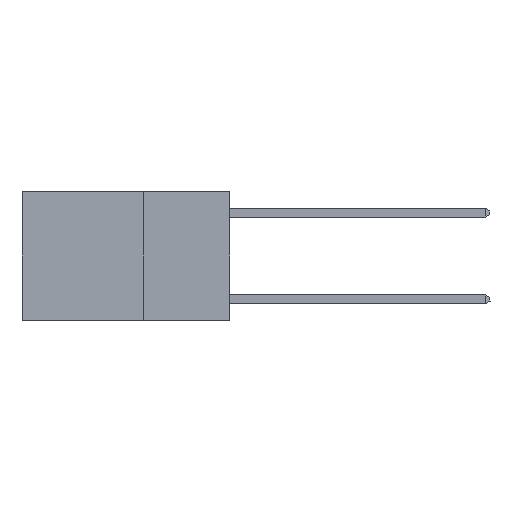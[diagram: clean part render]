
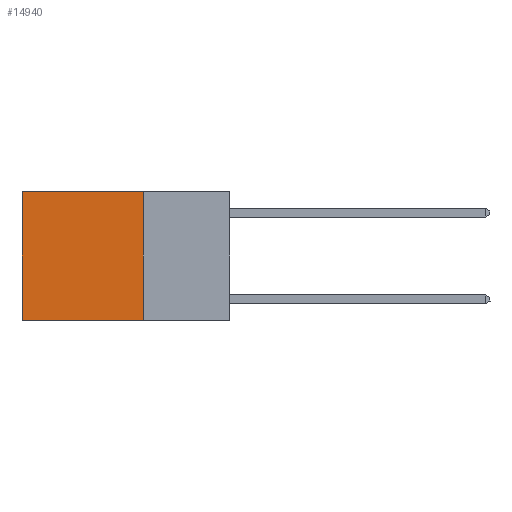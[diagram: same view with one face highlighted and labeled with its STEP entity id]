
A CAD part, left-side view. The second image highlights one B-rep face of the part: STEP entity #14940.
In plain terms, the highlighted planar face has unit normal (-1, 0, 0).
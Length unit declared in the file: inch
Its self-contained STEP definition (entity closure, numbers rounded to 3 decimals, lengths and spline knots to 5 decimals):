
#131 = DIRECTION ( 'NONE',  ( 0., 0., -1. ) ) ;
#175 = LINE ( 'NONE', #6093, #15766 ) ;
#477 = VERTEX_POINT ( 'NONE', #1827 ) ;
#612 = ORIENTED_EDGE ( 'NONE', *, *, #12786, .T. ) ;
#973 = DIRECTION ( 'NONE',  ( 0., 1., 0. ) ) ;
#1018 = CARTESIAN_POINT ( 'NONE',  ( 0.2625, 0.25, -0.37 ) ) ;
#1827 = CARTESIAN_POINT ( 'NONE',  ( 0.2625, 0.25, -0.37 ) ) ;
#1903 = CARTESIAN_POINT ( 'NONE',  ( 0.2625, 0.6, -0.37 ) ) ;
#3282 = VECTOR ( 'NONE', #8461, 39.37008 ) ;
#5583 = VECTOR ( 'NONE', #12988, 39.37008 ) ;
#6093 = CARTESIAN_POINT ( 'NONE',  ( 0.2625, 0.6, 0. ) ) ;
#6351 = LINE ( 'NONE', #17217, #3282 ) ;
#6955 = CARTESIAN_POINT ( 'NONE',  ( 0.2625, 0.25, 0. ) ) ;
#7615 = EDGE_CURVE ( 'NONE', #17538, #12568, #175, .T. ) ;
#8390 = FACE_OUTER_BOUND ( 'NONE', #15947, .T. ) ;
#8461 = DIRECTION ( 'NONE',  ( 0., 0., -1. ) ) ;
#9144 = DIRECTION ( 'NONE',  ( 1., 0., 0. ) ) ;
#10558 = DIRECTION ( 'NONE',  ( 0., 0., -1. ) ) ;
#11125 = AXIS2_PLACEMENT_3D ( 'NONE', #17877, #9144, #131 ) ;
#11266 = CARTESIAN_POINT ( 'NONE',  ( 0.2625, 0.6, 0. ) ) ;
#12539 = CARTESIAN_POINT ( 'NONE',  ( 0.2625, 0.25, 0. ) ) ;
#12568 = VERTEX_POINT ( 'NONE', #1903 ) ;
#12767 = EDGE_CURVE ( 'NONE', #13908, #477, #6351, .T. ) ;
#12786 = EDGE_CURVE ( 'NONE', #13908, #17538, #17582, .T. ) ;
#12988 = DIRECTION ( 'NONE',  ( 0., 1., 0. ) ) ;
#13308 = ORIENTED_EDGE ( 'NONE', *, *, #14676, .F. ) ;
#13735 = VECTOR ( 'NONE', #973, 39.37008 ) ;
#13801 = ORIENTED_EDGE ( 'NONE', *, *, #12767, .F. ) ;
#13908 = VERTEX_POINT ( 'NONE', #12539 ) ;
#14676 = EDGE_CURVE ( 'NONE', #477, #12568, #16399, .T. ) ;
#14940 = ADVANCED_FACE ( 'NONE', ( #8390 ), #14955, .F. ) ;
#14955 = PLANE ( 'NONE',  #11125 ) ;
#15617 = ORIENTED_EDGE ( 'NONE', *, *, #7615, .T. ) ;
#15766 = VECTOR ( 'NONE', #10558, 39.37008 ) ;
#15947 = EDGE_LOOP ( 'NONE', ( #15617, #13308, #13801, #612 ) ) ;
#16399 = LINE ( 'NONE', #1018, #5583 ) ;
#17217 = CARTESIAN_POINT ( 'NONE',  ( 0.2625, 0.25, 0. ) ) ;
#17538 = VERTEX_POINT ( 'NONE', #11266 ) ;
#17582 = LINE ( 'NONE', #6955, #13735 ) ;
#17877 = CARTESIAN_POINT ( 'NONE',  ( 0.2625, 0.25, 0. ) ) ;
